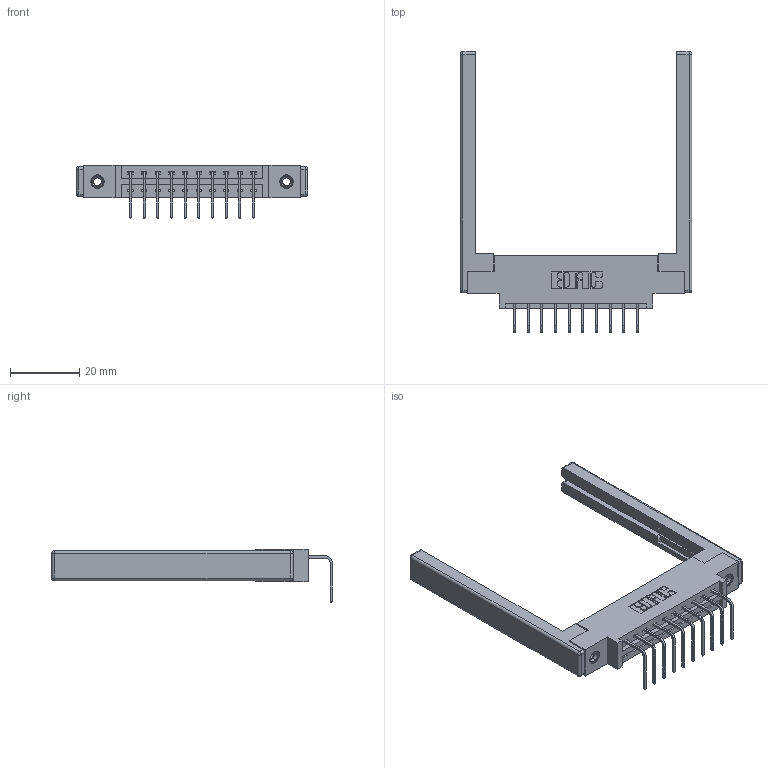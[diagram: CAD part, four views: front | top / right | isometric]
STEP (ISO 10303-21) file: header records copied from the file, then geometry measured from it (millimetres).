
FILE_DESCRIPTION (( 'STEP AP203' ), '1' );
FILE_NAME ('387-010-558-668.STEP', '2019-10-07T16:19:30', ( '' ), ( '' ), 'SwSTEP 2.0', 'SolidWorks 2016', '' );
FILE_SCHEMA (( 'CONFIG_CONTROL_DESIGN' ));
Length unit declared in the file: inch
Products named in the file (5): 345-250-001_345-250-001-102; 337 Part_0.170 Offset - 0.156 Dia-TI; 345-292-001_558 Tail - 2; 387-010-558-668; 307-220-068
Assembly tree (15 placements, depth 2):
  387-010-558-668
    337 Part_0.170 Offset - 0.156 Dia-TI
    345-292-001_558 Tail - 2  x10
    345-250-001_345-250-001-102  x2
    307-220-068  x2
Bounding box: 67.06 x 81.22 x 15.37 mm (x, y, z)
Volume: 10875.9 mm3; surface area: 10917.2 mm2
Topology: 15 solids, 15 shells, 912 faces, 2653 edges, 1734 vertices
Faces by surface type: plane 642, cylinder 246, cone 12, sphere 8, torus 4
Entity records: 14548 total; most frequent: CARTESIAN_POINT 2489, ORIENTED_EDGE 2424, DIRECTION 2234, EDGE_CURVE 1212, LINE 1034, VECTOR 1034, VERTEX_POINT 798, AXIS2_PLACEMENT_3D 600
